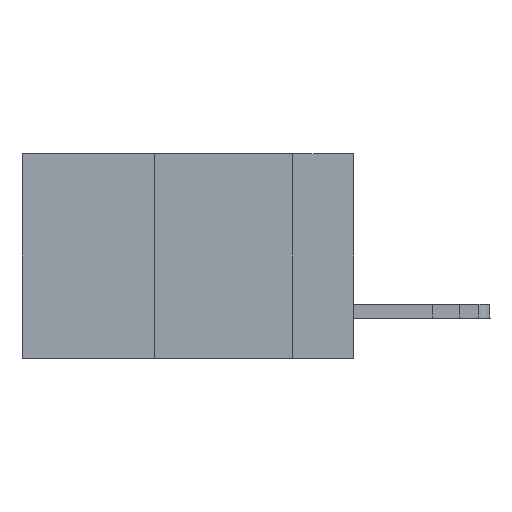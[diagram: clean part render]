
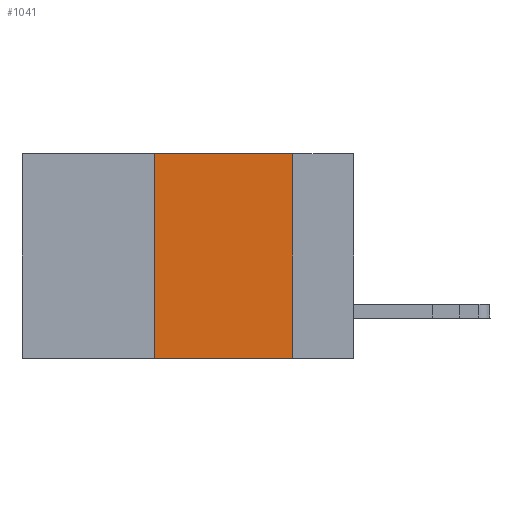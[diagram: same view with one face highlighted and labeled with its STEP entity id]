
A CAD part, left-side view. The second image highlights one B-rep face of the part: STEP entity #1041.
In plain terms, the highlighted planar face has unit normal (-1, 0, 0).
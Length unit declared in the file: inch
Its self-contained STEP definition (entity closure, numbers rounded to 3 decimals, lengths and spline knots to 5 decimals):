
#198 = ORIENTED_EDGE ( 'NONE', *, *, #13972, .F. ) ;
#237 = EDGE_CURVE ( 'NONE', #14014, #4762, #4027, .T. ) ;
#1019 = CARTESIAN_POINT ( 'NONE',  ( 0., 0.11, -0.37 ) ) ;
#1041 = ADVANCED_FACE ( 'NONE', ( #20095 ), #18409, .F. ) ;
#2504 = VECTOR ( 'NONE', #12808, 39.37008 ) ;
#2591 = LINE ( 'NONE', #8916, #3570 ) ;
#2893 = CARTESIAN_POINT ( 'NONE',  ( 0., 0.6, -0.37 ) ) ;
#3570 = VECTOR ( 'NONE', #13743, 39.37008 ) ;
#4027 = LINE ( 'NONE', #8306, #19395 ) ;
#4418 = DIRECTION ( 'NONE',  ( 0., 0., -1. ) ) ;
#4762 = VERTEX_POINT ( 'NONE', #1019 ) ;
#4787 = DIRECTION ( 'NONE',  ( 0., -1., 0. ) ) ;
#5045 = DIRECTION ( 'NONE',  ( 0., 0., -1. ) ) ;
#6714 = ORIENTED_EDGE ( 'NONE', *, *, #10505, .T. ) ;
#6824 = EDGE_LOOP ( 'NONE', ( #7686, #15885, #198, #6714 ) ) ;
#6941 = VERTEX_POINT ( 'NONE', #14372 ) ;
#7686 = ORIENTED_EDGE ( 'NONE', *, *, #237, .F. ) ;
#8306 = CARTESIAN_POINT ( 'NONE',  ( 0., 0.11, 0. ) ) ;
#8541 = AXIS2_PLACEMENT_3D ( 'NONE', #9129, #13875, #4418 ) ;
#8916 = CARTESIAN_POINT ( 'NONE',  ( 0., 0.6, 0. ) ) ;
#9129 = CARTESIAN_POINT ( 'NONE',  ( 0., 0.6, 0. ) ) ;
#10505 = EDGE_CURVE ( 'NONE', #13654, #4762, #19759, .T. ) ;
#10841 = VECTOR ( 'NONE', #4787, 39.37008 ) ;
#12808 = DIRECTION ( 'NONE',  ( 0., 0., 1. ) ) ;
#13319 = CARTESIAN_POINT ( 'NONE',  ( 0., 0.36, -0.37 ) ) ;
#13654 = VERTEX_POINT ( 'NONE', #13319 ) ;
#13743 = DIRECTION ( 'NONE',  ( 0., -1., 0. ) ) ;
#13875 = DIRECTION ( 'NONE',  ( 1., 0., 0. ) ) ;
#13972 = EDGE_CURVE ( 'NONE', #13654, #6941, #16336, .T. ) ;
#14014 = VERTEX_POINT ( 'NONE', #17610 ) ;
#14372 = CARTESIAN_POINT ( 'NONE',  ( 0., 0.36, 0. ) ) ;
#15858 = CARTESIAN_POINT ( 'NONE',  ( 0., 0.36, 0. ) ) ;
#15885 = ORIENTED_EDGE ( 'NONE', *, *, #18288, .F. ) ;
#16336 = LINE ( 'NONE', #15858, #2504 ) ;
#17610 = CARTESIAN_POINT ( 'NONE',  ( 0., 0.11, 0. ) ) ;
#18288 = EDGE_CURVE ( 'NONE', #6941, #14014, #2591, .T. ) ;
#18409 = PLANE ( 'NONE',  #8541 ) ;
#19395 = VECTOR ( 'NONE', #5045, 39.37008 ) ;
#19759 = LINE ( 'NONE', #2893, #10841 ) ;
#20095 = FACE_OUTER_BOUND ( 'NONE', #6824, .T. ) ;
